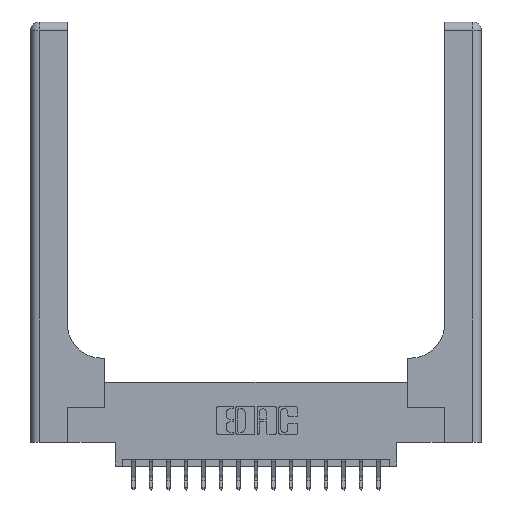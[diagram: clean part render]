
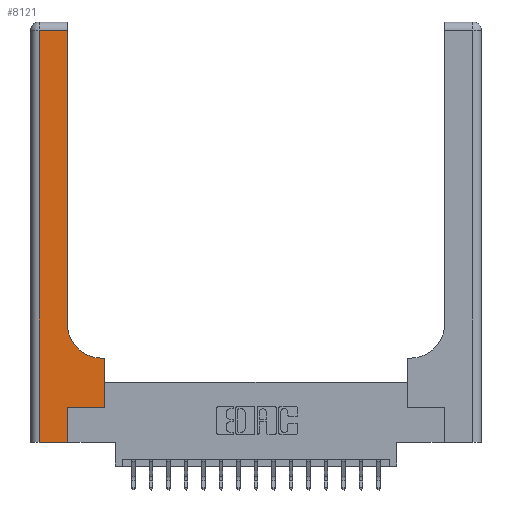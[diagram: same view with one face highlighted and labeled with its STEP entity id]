
A CAD part, top view. The second image highlights one B-rep face of the part: STEP entity #8121.
In plain terms, the highlighted planar face has unit normal (0, 0, 1).
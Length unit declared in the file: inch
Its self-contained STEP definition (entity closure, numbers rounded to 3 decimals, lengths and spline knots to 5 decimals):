
#10 = EDGE_CURVE ( 'NONE', #14892, #1073, #11088, .T. ) ;
#445 = VECTOR ( 'NONE', #18521, 39.37008 ) ;
#551 = VERTEX_POINT ( 'NONE', #10630 ) ;
#639 = LINE ( 'NONE', #15780, #12693 ) ;
#791 = CARTESIAN_POINT ( 'NONE',  ( 0.265, 0.25, 0.37 ) ) ;
#1073 = VERTEX_POINT ( 'NONE', #9977 ) ;
#1189 = CARTESIAN_POINT ( 'NONE',  ( 0.51, 0.6, 0.37 ) ) ;
#1228 = EDGE_CURVE ( 'NONE', #14557, #14892, #4815, .T. ) ;
#2433 = VERTEX_POINT ( 'NONE', #10449 ) ;
#3064 = CARTESIAN_POINT ( 'NONE',  ( 0.528, 0.25, 0.37 ) ) ;
#3184 = VERTEX_POINT ( 'NONE', #14175 ) ;
#3459 = VERTEX_POINT ( 'NONE', #10132 ) ;
#3632 = LINE ( 'NONE', #791, #10097 ) ;
#3700 = CIRCLE ( 'NONE', #5891, 0.25 ) ;
#3775 = LINE ( 'NONE', #9701, #19147 ) ;
#3793 = CARTESIAN_POINT ( 'NONE',  ( 0.06, 0., 0.37 ) ) ;
#3934 = DIRECTION ( 'NONE',  ( 1., 0., 0. ) ) ;
#4335 = DIRECTION ( 'NONE',  ( -1., 0., 0. ) ) ;
#4427 = DIRECTION ( 'NONE',  ( 0., 0., -1. ) ) ;
#4815 = LINE ( 'NONE', #9474, #8045 ) ;
#5019 = DIRECTION ( 'NONE',  ( -1., 0., 0. ) ) ;
#5854 = EDGE_LOOP ( 'NONE', ( #16703, #12010, #8421, #6642, #9103, #9909, #12530, #18785, #11847 ) ) ;
#5891 = AXIS2_PLACEMENT_3D ( 'NONE', #11420, #17399, #3934 ) ;
#6383 = EDGE_CURVE ( 'NONE', #3184, #8770, #639, .T. ) ;
#6388 = CARTESIAN_POINT ( 'NONE',  ( 0., 2.94, 0.37 ) ) ;
#6604 = VECTOR ( 'NONE', #13515, 39.37008 ) ;
#6642 = ORIENTED_EDGE ( 'NONE', *, *, #10, .T. ) ;
#6688 = LINE ( 'NONE', #6388, #14369 ) ;
#8045 = VECTOR ( 'NONE', #15256, 39.37008 ) ;
#8121 = ADVANCED_FACE ( 'NONE', ( #13394 ), #16050, .F. ) ;
#8192 = VERTEX_POINT ( 'NONE', #1189 ) ;
#8421 = ORIENTED_EDGE ( 'NONE', *, *, #1228, .T. ) ;
#8700 = CARTESIAN_POINT ( 'NONE',  ( 0.26, 0.6, 0.37 ) ) ;
#8770 = VERTEX_POINT ( 'NONE', #14843 ) ;
#9103 = ORIENTED_EDGE ( 'NONE', *, *, #16431, .T. ) ;
#9474 = CARTESIAN_POINT ( 'NONE',  ( 0.06, 3., 0.37 ) ) ;
#9701 = CARTESIAN_POINT ( 'NONE',  ( 0.265, 0., 0.37 ) ) ;
#9909 = ORIENTED_EDGE ( 'NONE', *, *, #17677, .T. ) ;
#9977 = CARTESIAN_POINT ( 'NONE',  ( 0.265, 0., 0.37 ) ) ;
#10097 = VECTOR ( 'NONE', #14178, 39.37008 ) ;
#10131 = CARTESIAN_POINT ( 'NONE',  ( 0.06, 2.94, 0.37 ) ) ;
#10132 = CARTESIAN_POINT ( 'NONE',  ( 0.528, 0.25, 0.37 ) ) ;
#10195 = EDGE_CURVE ( 'NONE', #8770, #14557, #6688, .T. ) ;
#10449 = CARTESIAN_POINT ( 'NONE',  ( 0.528, 0.6, 0.37 ) ) ;
#10630 = CARTESIAN_POINT ( 'NONE',  ( 0.265, 0.25, 0.37 ) ) ;
#11088 = LINE ( 'NONE', #15989, #445 ) ;
#11163 = EDGE_CURVE ( 'NONE', #2433, #8192, #19081, .T. ) ;
#11420 = CARTESIAN_POINT ( 'NONE',  ( 0.51, 0.85, 0.37 ) ) ;
#11633 = CARTESIAN_POINT ( 'NONE',  ( 0., 3., 0.37 ) ) ;
#11736 = EDGE_CURVE ( 'NONE', #8192, #3184, #3700, .T. ) ;
#11847 = ORIENTED_EDGE ( 'NONE', *, *, #11736, .T. ) ;
#12010 = ORIENTED_EDGE ( 'NONE', *, *, #10195, .T. ) ;
#12530 = ORIENTED_EDGE ( 'NONE', *, *, #18653, .T. ) ;
#12693 = VECTOR ( 'NONE', #18896, 39.37008 ) ;
#13394 = FACE_OUTER_BOUND ( 'NONE', #5854, .T. ) ;
#13442 = VECTOR ( 'NONE', #14877, 39.37008 ) ;
#13515 = DIRECTION ( 'NONE',  ( 0., 1., 0. ) ) ;
#14175 = CARTESIAN_POINT ( 'NONE',  ( 0.26, 0.85, 0.37 ) ) ;
#14178 = DIRECTION ( 'NONE',  ( 1., 0., 0. ) ) ;
#14369 = VECTOR ( 'NONE', #5019, 39.37008 ) ;
#14557 = VERTEX_POINT ( 'NONE', #10131 ) ;
#14843 = CARTESIAN_POINT ( 'NONE',  ( 0.26, 2.94, 0.37 ) ) ;
#14877 = DIRECTION ( 'NONE',  ( -1., 0., 0. ) ) ;
#14892 = VERTEX_POINT ( 'NONE', #3793 ) ;
#15256 = DIRECTION ( 'NONE',  ( 0., -1., 0. ) ) ;
#15277 = AXIS2_PLACEMENT_3D ( 'NONE', #11633, #4427, #4335 ) ;
#15780 = CARTESIAN_POINT ( 'NONE',  ( 0.26, 3., 0.37 ) ) ;
#15989 = CARTESIAN_POINT ( 'NONE',  ( 0., 0., 0.37 ) ) ;
#16050 = PLANE ( 'NONE',  #15277 ) ;
#16178 = LINE ( 'NONE', #3064, #6604 ) ;
#16431 = EDGE_CURVE ( 'NONE', #1073, #551, #3775, .T. ) ;
#16703 = ORIENTED_EDGE ( 'NONE', *, *, #6383, .T. ) ;
#17399 = DIRECTION ( 'NONE',  ( 0., 0., -1. ) ) ;
#17677 = EDGE_CURVE ( 'NONE', #551, #3459, #3632, .T. ) ;
#18521 = DIRECTION ( 'NONE',  ( 1., 0., 0. ) ) ;
#18653 = EDGE_CURVE ( 'NONE', #3459, #2433, #16178, .T. ) ;
#18785 = ORIENTED_EDGE ( 'NONE', *, *, #11163, .T. ) ;
#18896 = DIRECTION ( 'NONE',  ( 0., 1., 0. ) ) ;
#18997 = DIRECTION ( 'NONE',  ( 0., 1., 0. ) ) ;
#19081 = LINE ( 'NONE', #8700, #13442 ) ;
#19147 = VECTOR ( 'NONE', #18997, 39.37008 ) ;
